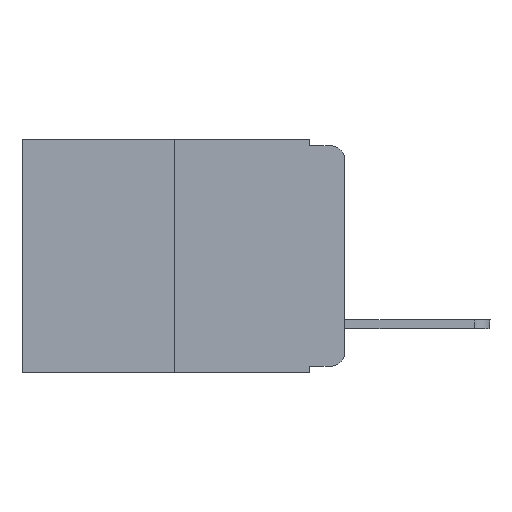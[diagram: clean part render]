
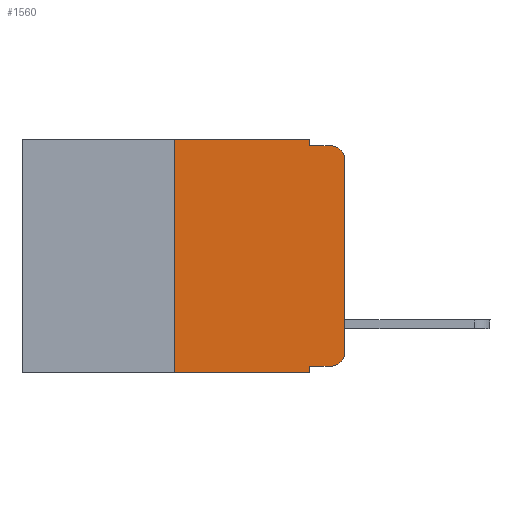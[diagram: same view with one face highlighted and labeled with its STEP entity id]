
A CAD part, left-side view. The second image highlights one B-rep face of the part: STEP entity #1560.
In plain terms, the highlighted planar face has unit normal (-1, 0, 0).
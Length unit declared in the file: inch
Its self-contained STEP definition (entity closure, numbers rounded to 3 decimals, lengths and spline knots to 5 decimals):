
#234 = DIRECTION ( 'NONE',  ( 0., 0., -1. ) ) ;
#412 = CARTESIAN_POINT ( 'NONE',  ( 0., 0.051, 0. ) ) ;
#429 = DIRECTION ( 'NONE',  ( 0., 0., 1. ) ) ;
#722 = VERTEX_POINT ( 'NONE', #2120 ) ;
#775 = CIRCLE ( 'NONE', #2511, 0.02 ) ;
#784 = ORIENTED_EDGE ( 'NONE', *, *, #9502, .T. ) ;
#831 = ORIENTED_EDGE ( 'NONE', *, *, #8132, .T. ) ;
#832 = DIRECTION ( 'NONE',  ( 0., -1., 0. ) ) ;
#1400 = ORIENTED_EDGE ( 'NONE', *, *, #4264, .T. ) ;
#1511 = CARTESIAN_POINT ( 'NONE',  ( 0., 0.25, 0. ) ) ;
#1560 = ADVANCED_FACE ( 'NONE', ( #10158 ), #3040, .F. ) ;
#1783 = ORIENTED_EDGE ( 'NONE', *, *, #12759, .T. ) ;
#1968 = VERTEX_POINT ( 'NONE', #10099 ) ;
#2120 = CARTESIAN_POINT ( 'NONE',  ( 0., 0.25, -0.343 ) ) ;
#2408 = DIRECTION ( 'NONE',  ( 0., 0., -1. ) ) ;
#2509 = LINE ( 'NONE', #10846, #14186 ) ;
#2511 = AXIS2_PLACEMENT_3D ( 'NONE', #12429, #14802, #2408 ) ;
#2880 = DIRECTION ( 'NONE',  ( 0., 0., -1. ) ) ;
#2896 = EDGE_LOOP ( 'NONE', ( #831, #784, #11374, #6742, #13014, #2976, #12473, #12077, #1783, #1400 ) ) ;
#2922 = CARTESIAN_POINT ( 'NONE',  ( 0., 0.02, -0.333 ) ) ;
#2976 = ORIENTED_EDGE ( 'NONE', *, *, #8443, .F. ) ;
#3040 = PLANE ( 'NONE',  #15094 ) ;
#3259 = CARTESIAN_POINT ( 'NONE',  ( 0., 0.473, 0. ) ) ;
#3374 = LINE ( 'NONE', #8275, #15465 ) ;
#3402 = VERTEX_POINT ( 'NONE', #2922 ) ;
#4245 = EDGE_CURVE ( 'NONE', #12270, #8230, #5234, .T. ) ;
#4264 = EDGE_CURVE ( 'NONE', #3402, #13722, #775, .T. ) ;
#4520 = DIRECTION ( 'NONE',  ( 0., 0., -1. ) ) ;
#5234 = LINE ( 'NONE', #3259, #14783 ) ;
#5252 = AXIS2_PLACEMENT_3D ( 'NONE', #13740, #6297, #234 ) ;
#5517 = CARTESIAN_POINT ( 'NONE',  ( 0., 0., -0.313 ) ) ;
#6297 = DIRECTION ( 'NONE',  ( -1., 0., 0. ) ) ;
#6531 = DIRECTION ( 'NONE',  ( 0., 0., -1. ) ) ;
#6731 = DIRECTION ( 'NONE',  ( 0., -1., 0. ) ) ;
#6742 = ORIENTED_EDGE ( 'NONE', *, *, #7645, .F. ) ;
#7517 = VECTOR ( 'NONE', #2880, 39.37008 ) ;
#7645 = EDGE_CURVE ( 'NONE', #8230, #9144, #15075, .T. ) ;
#7750 = DIRECTION ( 'NONE',  ( 0., -1., 0. ) ) ;
#8132 = EDGE_CURVE ( 'NONE', #13722, #14403, #15261, .T. ) ;
#8230 = VERTEX_POINT ( 'NONE', #15413 ) ;
#8275 = CARTESIAN_POINT ( 'NONE',  ( 0., 0.051, 0. ) ) ;
#8431 = CARTESIAN_POINT ( 'NONE',  ( 0., 0.051, -0.01 ) ) ;
#8443 = EDGE_CURVE ( 'NONE', #722, #12270, #14271, .T. ) ;
#8627 = VECTOR ( 'NONE', #7750, 39.37008 ) ;
#8886 = VECTOR ( 'NONE', #6731, 39.37008 ) ;
#9078 = EDGE_CURVE ( 'NONE', #13862, #1968, #3374, .T. ) ;
#9144 = VERTEX_POINT ( 'NONE', #8431 ) ;
#9463 = CARTESIAN_POINT ( 'NONE',  ( 0., 0.051, -0.01 ) ) ;
#9502 = EDGE_CURVE ( 'NONE', #14403, #15983, #11993, .T. ) ;
#10099 = CARTESIAN_POINT ( 'NONE',  ( 0., 0.051, -0.343 ) ) ;
#10158 = FACE_OUTER_BOUND ( 'NONE', #2896, .T. ) ;
#10224 = CARTESIAN_POINT ( 'NONE',  ( 0., 0.25, 0. ) ) ;
#10846 = CARTESIAN_POINT ( 'NONE',  ( 0., 0.051, -0.333 ) ) ;
#10950 = DIRECTION ( 'NONE',  ( 0., -1., 0. ) ) ;
#11184 = EDGE_CURVE ( 'NONE', #722, #1968, #12687, .T. ) ;
#11374 = ORIENTED_EDGE ( 'NONE', *, *, #16142, .F. ) ;
#11561 = VECTOR ( 'NONE', #14001, 39.37008 ) ;
#11764 = CARTESIAN_POINT ( 'NONE',  ( 0., 0.473, 0. ) ) ;
#11978 = VECTOR ( 'NONE', #429, 39.37008 ) ;
#11993 = CIRCLE ( 'NONE', #5252, 0.02 ) ;
#12077 = ORIENTED_EDGE ( 'NONE', *, *, #9078, .F. ) ;
#12179 = LINE ( 'NONE', #9463, #8886 ) ;
#12270 = VERTEX_POINT ( 'NONE', #10224 ) ;
#12429 = CARTESIAN_POINT ( 'NONE',  ( 0., 0.02, -0.313 ) ) ;
#12473 = ORIENTED_EDGE ( 'NONE', *, *, #11184, .T. ) ;
#12687 = LINE ( 'NONE', #13936, #8627 ) ;
#12759 = EDGE_CURVE ( 'NONE', #13862, #3402, #2509, .T. ) ;
#13014 = ORIENTED_EDGE ( 'NONE', *, *, #4245, .F. ) ;
#13673 = CARTESIAN_POINT ( 'NONE',  ( 0., 0.02, -0.01 ) ) ;
#13722 = VERTEX_POINT ( 'NONE', #5517 ) ;
#13740 = CARTESIAN_POINT ( 'NONE',  ( 0., 0.02, -0.03 ) ) ;
#13862 = VERTEX_POINT ( 'NONE', #15586 ) ;
#13936 = CARTESIAN_POINT ( 'NONE',  ( 0., 0.473, -0.343 ) ) ;
#13968 = DIRECTION ( 'NONE',  ( 1., 0., 0. ) ) ;
#14001 = DIRECTION ( 'NONE',  ( 0., 0., 1. ) ) ;
#14186 = VECTOR ( 'NONE', #10950, 39.37008 ) ;
#14271 = LINE ( 'NONE', #1511, #11561 ) ;
#14312 = CARTESIAN_POINT ( 'NONE',  ( 0., 0., -0.03 ) ) ;
#14403 = VERTEX_POINT ( 'NONE', #14312 ) ;
#14783 = VECTOR ( 'NONE', #832, 39.37008 ) ;
#14802 = DIRECTION ( 'NONE',  ( -1., 0., 0. ) ) ;
#15075 = LINE ( 'NONE', #412, #7517 ) ;
#15094 = AXIS2_PLACEMENT_3D ( 'NONE', #11764, #13968, #6531 ) ;
#15261 = LINE ( 'NONE', #15517, #11978 ) ;
#15413 = CARTESIAN_POINT ( 'NONE',  ( 0., 0.051, 0. ) ) ;
#15465 = VECTOR ( 'NONE', #4520, 39.37008 ) ;
#15517 = CARTESIAN_POINT ( 'NONE',  ( 0., 0., 0. ) ) ;
#15586 = CARTESIAN_POINT ( 'NONE',  ( 0., 0.051, -0.333 ) ) ;
#15983 = VERTEX_POINT ( 'NONE', #13673 ) ;
#16142 = EDGE_CURVE ( 'NONE', #9144, #15983, #12179, .T. ) ;
